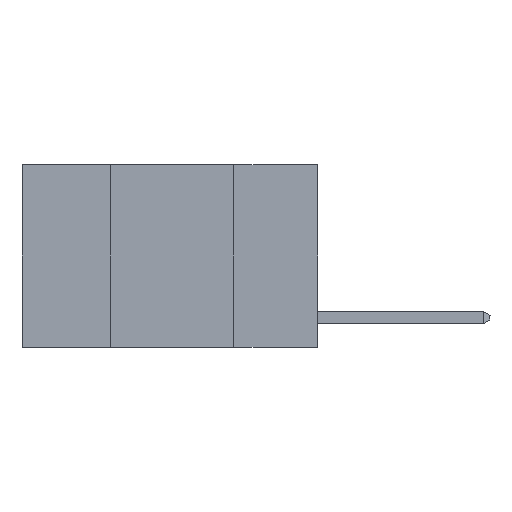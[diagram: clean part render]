
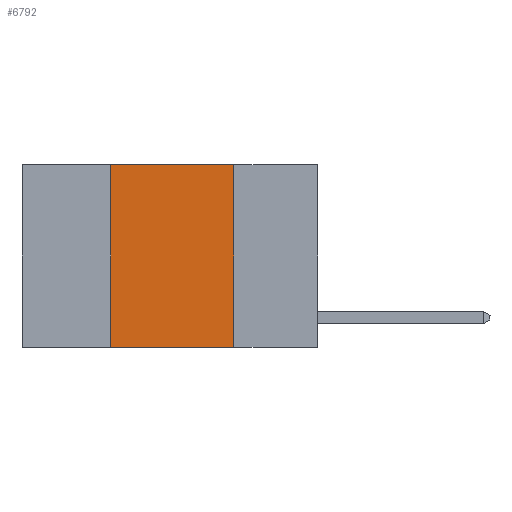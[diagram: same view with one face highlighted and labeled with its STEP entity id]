
A CAD part, left-side view. The second image highlights one B-rep face of the part: STEP entity #6792.
In plain terms, the highlighted planar face has unit normal (-1, 0, 0).
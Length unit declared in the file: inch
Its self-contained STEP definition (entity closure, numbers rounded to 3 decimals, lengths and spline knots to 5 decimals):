
#622 = ORIENTED_EDGE ( 'NONE', *, *, #11798, .F. ) ;
#912 = ORIENTED_EDGE ( 'NONE', *, *, #10310, .T. ) ;
#1493 = LINE ( 'NONE', #5345, #2813 ) ;
#1913 = CARTESIAN_POINT ( 'NONE',  ( 0., 0.42, -0.37 ) ) ;
#1994 = FACE_OUTER_BOUND ( 'NONE', #11169, .T. ) ;
#2297 = EDGE_CURVE ( 'NONE', #8651, #5854, #11115, .T. ) ;
#2663 = ORIENTED_EDGE ( 'NONE', *, *, #11616, .F. ) ;
#2813 = VECTOR ( 'NONE', #11109, 39.37008 ) ;
#3823 = LINE ( 'NONE', #8729, #5446 ) ;
#4255 = VERTEX_POINT ( 'NONE', #5353 ) ;
#4508 = CARTESIAN_POINT ( 'NONE',  ( 0., 0.17, 0. ) ) ;
#4589 = PLANE ( 'NONE',  #5282 ) ;
#4630 = LINE ( 'NONE', #4508, #9907 ) ;
#4819 = DIRECTION ( 'NONE',  ( 0., 0., 1. ) ) ;
#5282 = AXIS2_PLACEMENT_3D ( 'NONE', #10538, #12381, #8397 ) ;
#5345 = CARTESIAN_POINT ( 'NONE',  ( 0., 0.6, -0.37 ) ) ;
#5353 = CARTESIAN_POINT ( 'NONE',  ( 0., 0.17, -0.37 ) ) ;
#5446 = VECTOR ( 'NONE', #4819, 39.37008 ) ;
#5595 = DIRECTION ( 'NONE',  ( 0., -1., 0. ) ) ;
#5854 = VERTEX_POINT ( 'NONE', #8573 ) ;
#5965 = ORIENTED_EDGE ( 'NONE', *, *, #2297, .F. ) ;
#6792 = ADVANCED_FACE ( 'NONE', ( #1994 ), #4589, .F. ) ;
#8397 = DIRECTION ( 'NONE',  ( 0., 0., -1. ) ) ;
#8420 = VERTEX_POINT ( 'NONE', #1913 ) ;
#8573 = CARTESIAN_POINT ( 'NONE',  ( 0., 0.17, 0. ) ) ;
#8648 = VECTOR ( 'NONE', #5595, 39.37008 ) ;
#8651 = VERTEX_POINT ( 'NONE', #11875 ) ;
#8729 = CARTESIAN_POINT ( 'NONE',  ( 0., 0.42, 0. ) ) ;
#9907 = VECTOR ( 'NONE', #11205, 39.37008 ) ;
#10310 = EDGE_CURVE ( 'NONE', #8420, #4255, #1493, .T. ) ;
#10538 = CARTESIAN_POINT ( 'NONE',  ( 0., 0.6, 0. ) ) ;
#11109 = DIRECTION ( 'NONE',  ( 0., -1., 0. ) ) ;
#11115 = LINE ( 'NONE', #12207, #8648 ) ;
#11169 = EDGE_LOOP ( 'NONE', ( #2663, #5965, #622, #912 ) ) ;
#11205 = DIRECTION ( 'NONE',  ( 0., 0., -1. ) ) ;
#11616 = EDGE_CURVE ( 'NONE', #5854, #4255, #4630, .T. ) ;
#11798 = EDGE_CURVE ( 'NONE', #8420, #8651, #3823, .T. ) ;
#11875 = CARTESIAN_POINT ( 'NONE',  ( 0., 0.42, 0. ) ) ;
#12207 = CARTESIAN_POINT ( 'NONE',  ( 0., 0.6, 0. ) ) ;
#12381 = DIRECTION ( 'NONE',  ( 1., 0., 0. ) ) ;
